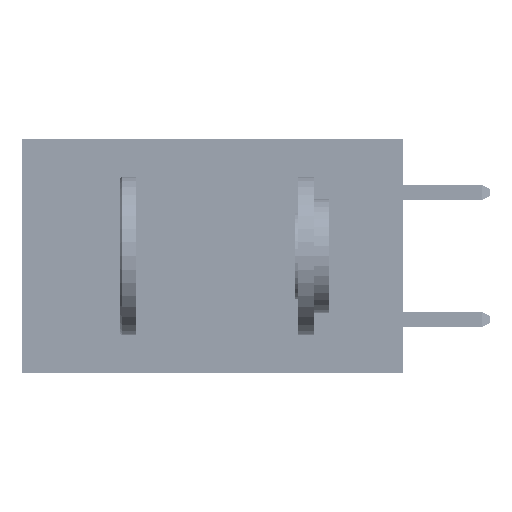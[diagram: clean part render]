
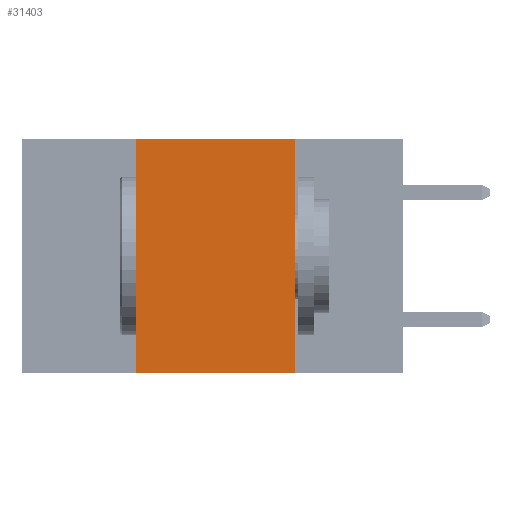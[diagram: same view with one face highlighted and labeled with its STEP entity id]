
A CAD part, left-side view. The second image highlights one B-rep face of the part: STEP entity #31403.
In plain terms, the highlighted planar face has unit normal (-1, 0, 0).
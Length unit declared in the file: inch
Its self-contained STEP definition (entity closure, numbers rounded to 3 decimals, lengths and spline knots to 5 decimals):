
#16 = CARTESIAN_POINT ( 'NONE',  ( 0., 0.17, 0. ) ) ;
#618 = EDGE_CURVE ( 'NONE', #3851, #37562, #1022, .T. ) ;
#1022 = LINE ( 'NONE', #22980, #26135 ) ;
#2810 = DIRECTION ( 'NONE',  ( 0., 0., 1. ) ) ;
#3851 = VERTEX_POINT ( 'NONE', #17128 ) ;
#4378 = VERTEX_POINT ( 'NONE', #44900 ) ;
#4492 = EDGE_LOOP ( 'NONE', ( #44543, #26037, #49266, #29509 ) ) ;
#4887 = AXIS2_PLACEMENT_3D ( 'NONE', #21225, #41228, #45257 ) ;
#7797 = DIRECTION ( 'NONE',  ( 0., -1., 0. ) ) ;
#9132 = PLANE ( 'NONE',  #4887 ) ;
#13417 = LINE ( 'NONE', #32949, #42274 ) ;
#16868 = VECTOR ( 'NONE', #7797, 39.37008 ) ;
#17128 = CARTESIAN_POINT ( 'NONE',  ( 0., 0.42, -0.37 ) ) ;
#19731 = CARTESIAN_POINT ( 'NONE',  ( 0., 0.6, 0. ) ) ;
#21225 = CARTESIAN_POINT ( 'NONE',  ( 0., 0.6, 0. ) ) ;
#22980 = CARTESIAN_POINT ( 'NONE',  ( 0., 0.42, 0. ) ) ;
#23260 = CARTESIAN_POINT ( 'NONE',  ( 0., 0.17, 0. ) ) ;
#25778 = VERTEX_POINT ( 'NONE', #16 ) ;
#26037 = ORIENTED_EDGE ( 'NONE', *, *, #43523, .F. ) ;
#26135 = VECTOR ( 'NONE', #2810, 39.37008 ) ;
#27558 = VECTOR ( 'NONE', #51498, 39.37008 ) ;
#29509 = ORIENTED_EDGE ( 'NONE', *, *, #45877, .T. ) ;
#31403 = ADVANCED_FACE ( 'NONE', ( #47574 ), #9132, .F. ) ;
#32949 = CARTESIAN_POINT ( 'NONE',  ( 0., 0.6, -0.37 ) ) ;
#36266 = EDGE_CURVE ( 'NONE', #25778, #4378, #49516, .T. ) ;
#37562 = VERTEX_POINT ( 'NONE', #39945 ) ;
#38187 = LINE ( 'NONE', #19731, #16868 ) ;
#39945 = CARTESIAN_POINT ( 'NONE',  ( 0., 0.42, 0. ) ) ;
#41002 = DIRECTION ( 'NONE',  ( 0., -1., 0. ) ) ;
#41228 = DIRECTION ( 'NONE',  ( 1., 0., 0. ) ) ;
#42274 = VECTOR ( 'NONE', #41002, 39.37008 ) ;
#43523 = EDGE_CURVE ( 'NONE', #37562, #25778, #38187, .T. ) ;
#44543 = ORIENTED_EDGE ( 'NONE', *, *, #36266, .F. ) ;
#44900 = CARTESIAN_POINT ( 'NONE',  ( 0., 0.17, -0.37 ) ) ;
#45257 = DIRECTION ( 'NONE',  ( 0., 0., -1. ) ) ;
#45877 = EDGE_CURVE ( 'NONE', #3851, #4378, #13417, .T. ) ;
#47574 = FACE_OUTER_BOUND ( 'NONE', #4492, .T. ) ;
#49266 = ORIENTED_EDGE ( 'NONE', *, *, #618, .F. ) ;
#49516 = LINE ( 'NONE', #23260, #27558 ) ;
#51498 = DIRECTION ( 'NONE',  ( 0., 0., -1. ) ) ;
